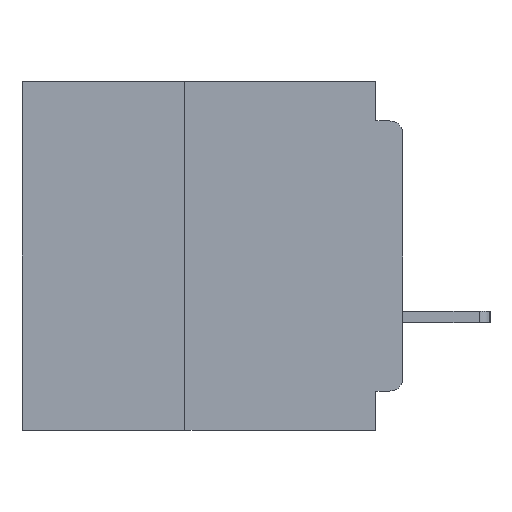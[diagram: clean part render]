
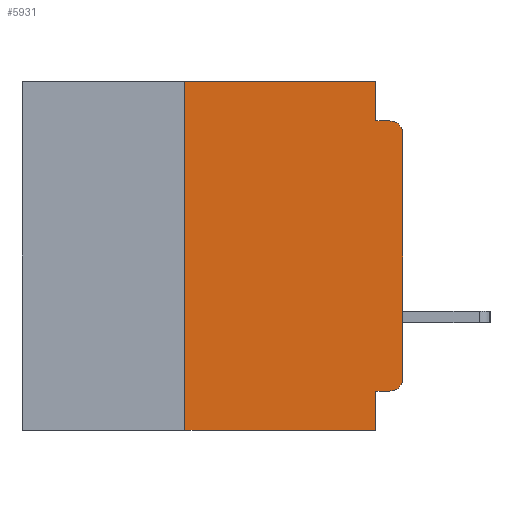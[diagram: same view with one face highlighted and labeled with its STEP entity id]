
A CAD part, left-side view. The second image highlights one B-rep face of the part: STEP entity #5931.
In plain terms, the highlighted planar face has unit normal (-1, 0, 0).
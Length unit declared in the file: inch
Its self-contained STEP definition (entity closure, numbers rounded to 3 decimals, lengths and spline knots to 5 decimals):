
#400 = VECTOR ( 'NONE', #29474, 39.37008 ) ;
#550 = CARTESIAN_POINT ( 'NONE',  ( 0., 0., -0.06 ) ) ;
#1224 = VERTEX_POINT ( 'NONE', #32519 ) ;
#1331 = CARTESIAN_POINT ( 'NONE',  ( 0., 0.015, -0.34 ) ) ;
#1619 = CARTESIAN_POINT ( 'NONE',  ( 0., 0.031, 0. ) ) ;
#1816 = DIRECTION ( 'NONE',  ( 0., 0., 1. ) ) ;
#1915 = VERTEX_POINT ( 'NONE', #28077 ) ;
#2474 = EDGE_CURVE ( 'NONE', #20168, #28548, #29622, .T. ) ;
#2717 = DIRECTION ( 'NONE',  ( 0., -1., 0. ) ) ;
#4461 = DIRECTION ( 'NONE',  ( 0., 0., -1. ) ) ;
#4664 = ORIENTED_EDGE ( 'NONE', *, *, #20785, .T. ) ;
#4739 = PLANE ( 'NONE',  #39075 ) ;
#4853 = DIRECTION ( 'NONE',  ( 0., -1., 0. ) ) ;
#5609 = VECTOR ( 'NONE', #4853, 39.37008 ) ;
#5737 = LINE ( 'NONE', #14276, #400 ) ;
#5931 = ADVANCED_FACE ( 'NONE', ( #10519 ), #4739, .F. ) ;
#7031 = VECTOR ( 'NONE', #17996, 39.37008 ) ;
#7607 = CARTESIAN_POINT ( 'NONE',  ( 0., 0.031, -0.355 ) ) ;
#7713 = EDGE_CURVE ( 'NONE', #12675, #20021, #29921, .T. ) ;
#7828 = DIRECTION ( 'NONE',  ( 0., 0., -1. ) ) ;
#7881 = EDGE_CURVE ( 'NONE', #28548, #1224, #23172, .T. ) ;
#8214 = CARTESIAN_POINT ( 'NONE',  ( 0., 0.015, -0.355 ) ) ;
#8296 = DIRECTION ( 'NONE',  ( -1., 0., 0. ) ) ;
#8973 = VERTEX_POINT ( 'NONE', #23117 ) ;
#9452 = ORIENTED_EDGE ( 'NONE', *, *, #24044, .F. ) ;
#9927 = ORIENTED_EDGE ( 'NONE', *, *, #14277, .T. ) ;
#10519 = FACE_OUTER_BOUND ( 'NONE', #15603, .T. ) ;
#11223 = VERTEX_POINT ( 'NONE', #26235 ) ;
#11538 = DIRECTION ( 'NONE',  ( 0., -1., 0. ) ) ;
#11904 = EDGE_CURVE ( 'NONE', #8973, #1224, #30506, .T. ) ;
#12341 = ORIENTED_EDGE ( 'NONE', *, *, #2474, .F. ) ;
#12459 = CARTESIAN_POINT ( 'NONE',  ( 0., 0.25, 0. ) ) ;
#12621 = LINE ( 'NONE', #17041, #19710 ) ;
#12675 = VERTEX_POINT ( 'NONE', #12459 ) ;
#13831 = CARTESIAN_POINT ( 'NONE',  ( 0., 0.437, 0. ) ) ;
#14066 = CARTESIAN_POINT ( 'NONE',  ( 0., 0.25, -0.4 ) ) ;
#14276 = CARTESIAN_POINT ( 'NONE',  ( 0., 0.031, 0. ) ) ;
#14277 = EDGE_CURVE ( 'NONE', #1915, #36257, #12621, .T. ) ;
#15603 = EDGE_LOOP ( 'NONE', ( #9927, #4664, #20860, #37932, #22755, #9452, #25641, #35577, #12341, #37476 ) ) ;
#16257 = VECTOR ( 'NONE', #20148, 39.37008 ) ;
#17041 = CARTESIAN_POINT ( 'NONE',  ( 0., 0., 0. ) ) ;
#17880 = EDGE_CURVE ( 'NONE', #20021, #11223, #5737, .T. ) ;
#17996 = DIRECTION ( 'NONE',  ( 0., 0., -1. ) ) ;
#19710 = VECTOR ( 'NONE', #1816, 39.37008 ) ;
#20021 = VERTEX_POINT ( 'NONE', #1619 ) ;
#20148 = DIRECTION ( 'NONE',  ( 0., 0., 1. ) ) ;
#20168 = VERTEX_POINT ( 'NONE', #8214 ) ;
#20785 = EDGE_CURVE ( 'NONE', #36257, #31898, #36933, .T. ) ;
#20860 = ORIENTED_EDGE ( 'NONE', *, *, #31676, .F. ) ;
#20991 = CARTESIAN_POINT ( 'NONE',  ( 0., 0.437, -0.4 ) ) ;
#22343 = VECTOR ( 'NONE', #2717, 39.37008 ) ;
#22678 = DIRECTION ( 'NONE',  ( -1., 0., 0. ) ) ;
#22755 = ORIENTED_EDGE ( 'NONE', *, *, #7713, .F. ) ;
#23117 = CARTESIAN_POINT ( 'NONE',  ( 0., 0.25, -0.4 ) ) ;
#23172 = LINE ( 'NONE', #24110, #7031 ) ;
#24044 = EDGE_CURVE ( 'NONE', #8973, #12675, #32442, .T. ) ;
#24110 = CARTESIAN_POINT ( 'NONE',  ( 0., 0.031, -0.4 ) ) ;
#25041 = AXIS2_PLACEMENT_3D ( 'NONE', #1331, #22678, #4461 ) ;
#25641 = ORIENTED_EDGE ( 'NONE', *, *, #11904, .T. ) ;
#25979 = AXIS2_PLACEMENT_3D ( 'NONE', #26528, #8296, #29614 ) ;
#26046 = DIRECTION ( 'NONE',  ( 1., 0., 0. ) ) ;
#26235 = CARTESIAN_POINT ( 'NONE',  ( 0., 0.031, -0.045 ) ) ;
#26299 = CARTESIAN_POINT ( 'NONE',  ( 0., 0.437, 0. ) ) ;
#26528 = CARTESIAN_POINT ( 'NONE',  ( 0., 0.015, -0.06 ) ) ;
#28077 = CARTESIAN_POINT ( 'NONE',  ( 0., 0., -0.34 ) ) ;
#28548 = VERTEX_POINT ( 'NONE', #7607 ) ;
#29474 = DIRECTION ( 'NONE',  ( 0., 0., -1. ) ) ;
#29614 = DIRECTION ( 'NONE',  ( 0., 0., -1. ) ) ;
#29622 = LINE ( 'NONE', #37394, #37599 ) ;
#29717 = EDGE_CURVE ( 'NONE', #20168, #1915, #35614, .T. ) ;
#29921 = LINE ( 'NONE', #26299, #5609 ) ;
#30506 = LINE ( 'NONE', #20991, #22343 ) ;
#31676 = EDGE_CURVE ( 'NONE', #11223, #31898, #35923, .T. ) ;
#31898 = VERTEX_POINT ( 'NONE', #33969 ) ;
#32442 = LINE ( 'NONE', #14066, #16257 ) ;
#32496 = DIRECTION ( 'NONE',  ( 0., 1., 0. ) ) ;
#32519 = CARTESIAN_POINT ( 'NONE',  ( 0., 0.031, -0.4 ) ) ;
#32797 = CARTESIAN_POINT ( 'NONE',  ( 0., 0., -0.045 ) ) ;
#33969 = CARTESIAN_POINT ( 'NONE',  ( 0., 0.015, -0.045 ) ) ;
#34981 = VECTOR ( 'NONE', #11538, 39.37008 ) ;
#35577 = ORIENTED_EDGE ( 'NONE', *, *, #7881, .F. ) ;
#35614 = CIRCLE ( 'NONE', #25041, 0.015 ) ;
#35923 = LINE ( 'NONE', #32797, #34981 ) ;
#36257 = VERTEX_POINT ( 'NONE', #550 ) ;
#36933 = CIRCLE ( 'NONE', #25979, 0.015 ) ;
#37394 = CARTESIAN_POINT ( 'NONE',  ( 0., 0., -0.355 ) ) ;
#37476 = ORIENTED_EDGE ( 'NONE', *, *, #29717, .T. ) ;
#37599 = VECTOR ( 'NONE', #32496, 39.37008 ) ;
#37932 = ORIENTED_EDGE ( 'NONE', *, *, #17880, .F. ) ;
#39075 = AXIS2_PLACEMENT_3D ( 'NONE', #13831, #26046, #7828 ) ;
